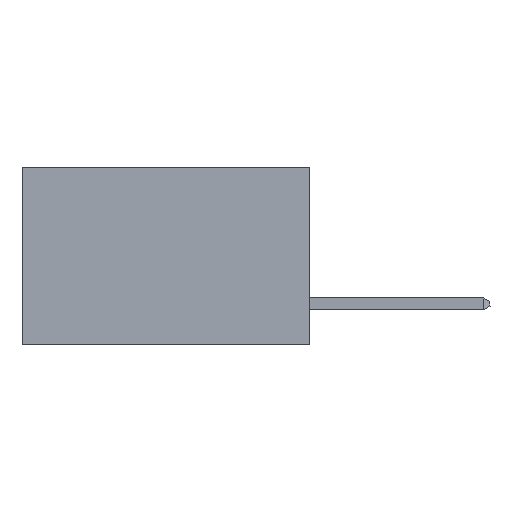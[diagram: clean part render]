
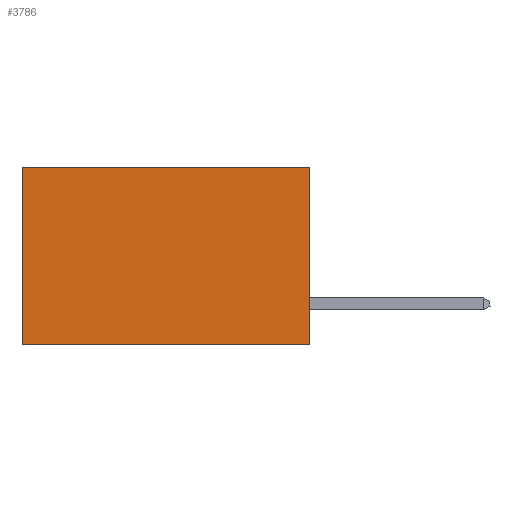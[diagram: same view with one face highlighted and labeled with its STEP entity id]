
A CAD part, left-side view. The second image highlights one B-rep face of the part: STEP entity #3786.
In plain terms, the highlighted planar face has unit normal (-1, 0, 0).
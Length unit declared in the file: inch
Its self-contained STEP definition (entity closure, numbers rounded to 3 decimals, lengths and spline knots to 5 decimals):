
#521 = ORIENTED_EDGE ( 'NONE', *, *, #22691, .T. ) ;
#922 = VERTEX_POINT ( 'NONE', #17572 ) ;
#1326 = EDGE_CURVE ( 'NONE', #20182, #6784, #13238, .T. ) ;
#1613 = ORIENTED_EDGE ( 'NONE', *, *, #11398, .F. ) ;
#1679 = LINE ( 'NONE', #4345, #20691 ) ;
#1825 = CARTESIAN_POINT ( 'NONE',  ( 0.2875, 0., 0. ) ) ;
#2172 = CARTESIAN_POINT ( 'NONE',  ( 0.2875, 0., 0. ) ) ;
#3786 = ADVANCED_FACE ( 'NONE', ( #7187 ), #18712, .F. ) ;
#3820 = DIRECTION ( 'NONE',  ( 0., 1., 0. ) ) ;
#4345 = CARTESIAN_POINT ( 'NONE',  ( 0.2875, 0., -0.37 ) ) ;
#5155 = VECTOR ( 'NONE', #22226, 39.37008 ) ;
#5333 = CARTESIAN_POINT ( 'NONE',  ( 0.2875, 0., 0. ) ) ;
#5795 = ORIENTED_EDGE ( 'NONE', *, *, #19456, .F. ) ;
#6146 = CARTESIAN_POINT ( 'NONE',  ( 0.2875, 0.6, 0. ) ) ;
#6292 = DIRECTION ( 'NONE',  ( 0., 1., 0. ) ) ;
#6784 = VERTEX_POINT ( 'NONE', #6146 ) ;
#7187 = FACE_OUTER_BOUND ( 'NONE', #14762, .T. ) ;
#8231 = VECTOR ( 'NONE', #3820, 39.37008 ) ;
#8810 = DIRECTION ( 'NONE',  ( 0., 0., -1. ) ) ;
#11145 = AXIS2_PLACEMENT_3D ( 'NONE', #2172, #15044, #8810 ) ;
#11398 = EDGE_CURVE ( 'NONE', #922, #11855, #1679, .T. ) ;
#11535 = CARTESIAN_POINT ( 'NONE',  ( 0.2875, 0., 0. ) ) ;
#11855 = VERTEX_POINT ( 'NONE', #15207 ) ;
#13238 = LINE ( 'NONE', #5333, #8231 ) ;
#14481 = ORIENTED_EDGE ( 'NONE', *, *, #1326, .T. ) ;
#14762 = EDGE_LOOP ( 'NONE', ( #521, #1613, #5795, #14481 ) ) ;
#15044 = DIRECTION ( 'NONE',  ( 1., 0., 0. ) ) ;
#15203 = DIRECTION ( 'NONE',  ( 0., 0., -1. ) ) ;
#15207 = CARTESIAN_POINT ( 'NONE',  ( 0.2875, 0.6, -0.37 ) ) ;
#17572 = CARTESIAN_POINT ( 'NONE',  ( 0.2875, 0., -0.37 ) ) ;
#18038 = LINE ( 'NONE', #1825, #23561 ) ;
#18712 = PLANE ( 'NONE',  #11145 ) ;
#19456 = EDGE_CURVE ( 'NONE', #20182, #922, #18038, .T. ) ;
#20182 = VERTEX_POINT ( 'NONE', #11535 ) ;
#20225 = LINE ( 'NONE', #20355, #5155 ) ;
#20355 = CARTESIAN_POINT ( 'NONE',  ( 0.2875, 0.6, 0. ) ) ;
#20691 = VECTOR ( 'NONE', #6292, 39.37008 ) ;
#22226 = DIRECTION ( 'NONE',  ( 0., 0., -1. ) ) ;
#22691 = EDGE_CURVE ( 'NONE', #6784, #11855, #20225, .T. ) ;
#23561 = VECTOR ( 'NONE', #15203, 39.37008 ) ;
